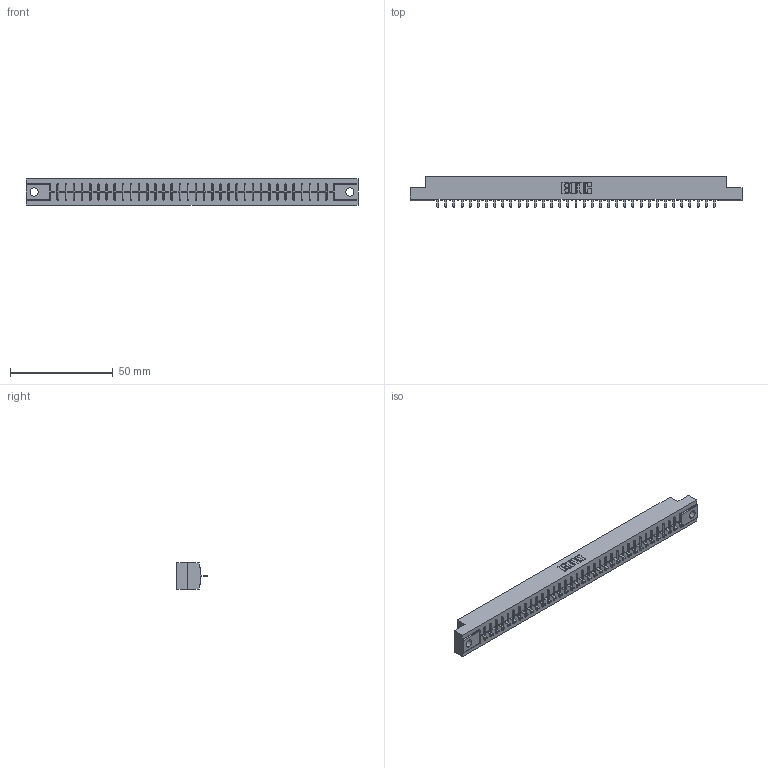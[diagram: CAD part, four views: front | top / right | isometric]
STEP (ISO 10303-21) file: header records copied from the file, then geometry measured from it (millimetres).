
FILE_DESCRIPTION (( 'STEP AP203' ), '1' );
FILE_NAME ('306-035-421-104.STEP', '2020-09-22T04:03:31', ( '' ), ( '' ), 'SwSTEP 2.0', 'SolidWorks 2020', '' );
FILE_SCHEMA (( 'CONFIG_CONTROL_DESIGN' ));
Length unit declared in the file: inch
Products named in the file (3): 306-290-001_121; 306 Part_.156 Dia; 306-035-421-104
Assembly tree (36 placements, depth 2):
  306-035-421-104
    306 Part_.156 Dia
    306-290-001_121  x35
Bounding box: 161.7 x 14.88 x 12.7 mm (x, y, z)
Volume: 17665.4 mm3; surface area: 17621.3 mm2
Topology: 36 solids, 36 shells, 2580 faces, 7247 edges, 4642 vertices
Faces by surface type: plane 1727, cylinder 713, sphere 140
Entity records: 33920 total; most frequent: CARTESIAN_POINT 5698, ORIENTED_EDGE 5646, DIRECTION 5611, EDGE_CURVE 2823, LINE 2213, VECTOR 2213, VERTEX_POINT 1786, AXIS2_PLACEMENT_3D 1699
